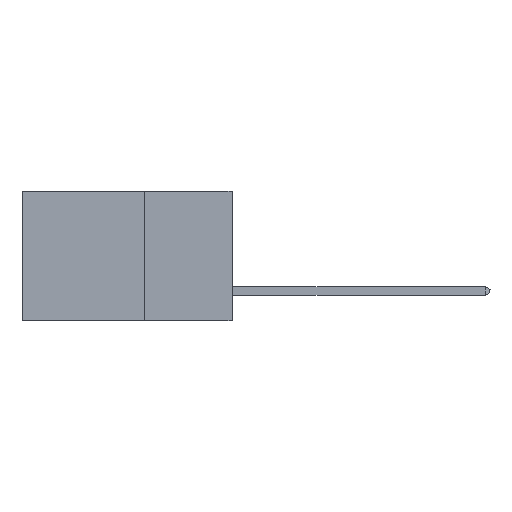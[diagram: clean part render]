
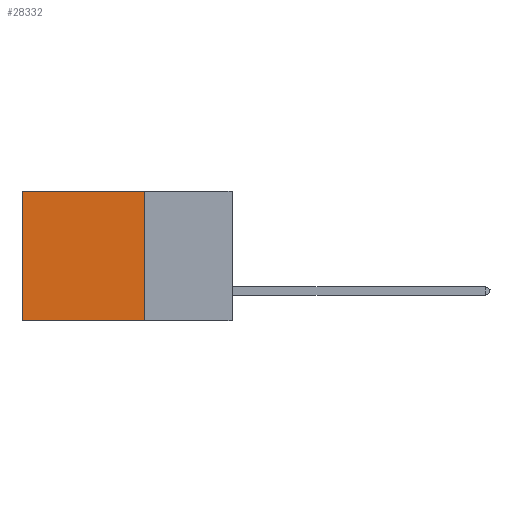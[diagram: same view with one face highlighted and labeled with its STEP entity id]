
A CAD part, left-side view. The second image highlights one B-rep face of the part: STEP entity #28332.
In plain terms, the highlighted planar face has unit normal (-1, 0, 0).
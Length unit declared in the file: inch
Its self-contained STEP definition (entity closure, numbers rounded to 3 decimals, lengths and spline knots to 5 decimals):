
#41 = CARTESIAN_POINT ( 'NONE',  ( 0.2875, 0.25, -0.37 ) ) ;
#695 = PLANE ( 'NONE',  #17588 ) ;
#2284 = CARTESIAN_POINT ( 'NONE',  ( 0.2875, 0.25, 0. ) ) ;
#2641 = EDGE_CURVE ( 'NONE', #8207, #3875, #28159, .T. ) ;
#2695 = ORIENTED_EDGE ( 'NONE', *, *, #18409, .F. ) ;
#2702 = CARTESIAN_POINT ( 'NONE',  ( 0.2875, 0.25, 0. ) ) ;
#3875 = VERTEX_POINT ( 'NONE', #4588 ) ;
#4588 = CARTESIAN_POINT ( 'NONE',  ( 0.2875, 0.6, -0.37 ) ) ;
#4996 = VERTEX_POINT ( 'NONE', #41 ) ;
#5007 = FACE_OUTER_BOUND ( 'NONE', #12565, .T. ) ;
#6930 = ORIENTED_EDGE ( 'NONE', *, *, #13519, .F. ) ;
#7668 = DIRECTION ( 'NONE',  ( 0., 0., -1. ) ) ;
#8155 = CARTESIAN_POINT ( 'NONE',  ( 0.2875, 0.25, 0. ) ) ;
#8207 = VERTEX_POINT ( 'NONE', #25116 ) ;
#9509 = ORIENTED_EDGE ( 'NONE', *, *, #11560, .T. ) ;
#10838 = DIRECTION ( 'NONE',  ( 0., 0., -1. ) ) ;
#11353 = DIRECTION ( 'NONE',  ( 0., 0., -1. ) ) ;
#11560 = EDGE_CURVE ( 'NONE', #12930, #8207, #21094, .T. ) ;
#12565 = EDGE_LOOP ( 'NONE', ( #26404, #6930, #2695, #9509 ) ) ;
#12930 = VERTEX_POINT ( 'NONE', #2702 ) ;
#13519 = EDGE_CURVE ( 'NONE', #4996, #3875, #23570, .T. ) ;
#15706 = VECTOR ( 'NONE', #11353, 39.37008 ) ;
#15884 = DIRECTION ( 'NONE',  ( 0., 1., 0. ) ) ;
#17101 = DIRECTION ( 'NONE',  ( 1., 0., 0. ) ) ;
#17588 = AXIS2_PLACEMENT_3D ( 'NONE', #19238, #17101, #7668 ) ;
#17788 = LINE ( 'NONE', #8155, #19979 ) ;
#18170 = VECTOR ( 'NONE', #23300, 39.37008 ) ;
#18409 = EDGE_CURVE ( 'NONE', #12930, #4996, #17788, .T. ) ;
#19238 = CARTESIAN_POINT ( 'NONE',  ( 0.2875, 0.25, 0. ) ) ;
#19979 = VECTOR ( 'NONE', #10838, 39.37008 ) ;
#20284 = VECTOR ( 'NONE', #15884, 39.37008 ) ;
#21094 = LINE ( 'NONE', #2284, #18170 ) ;
#23300 = DIRECTION ( 'NONE',  ( 0., 1., 0. ) ) ;
#23462 = CARTESIAN_POINT ( 'NONE',  ( 0.2875, 0.6, 0. ) ) ;
#23570 = LINE ( 'NONE', #24363, #20284 ) ;
#24363 = CARTESIAN_POINT ( 'NONE',  ( 0.2875, 0.25, -0.37 ) ) ;
#25116 = CARTESIAN_POINT ( 'NONE',  ( 0.2875, 0.6, 0. ) ) ;
#26404 = ORIENTED_EDGE ( 'NONE', *, *, #2641, .T. ) ;
#28159 = LINE ( 'NONE', #23462, #15706 ) ;
#28332 = ADVANCED_FACE ( 'NONE', ( #5007 ), #695, .F. ) ;
